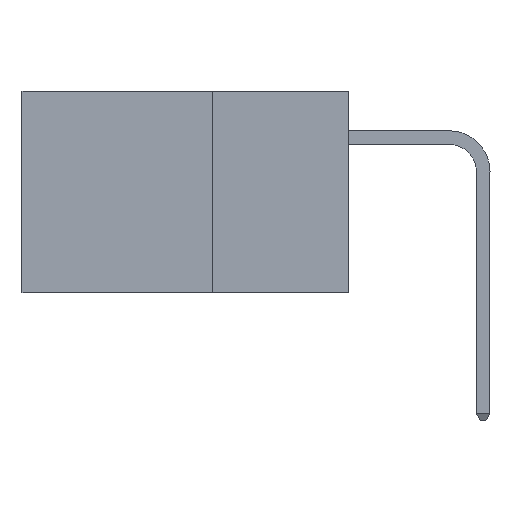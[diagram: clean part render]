
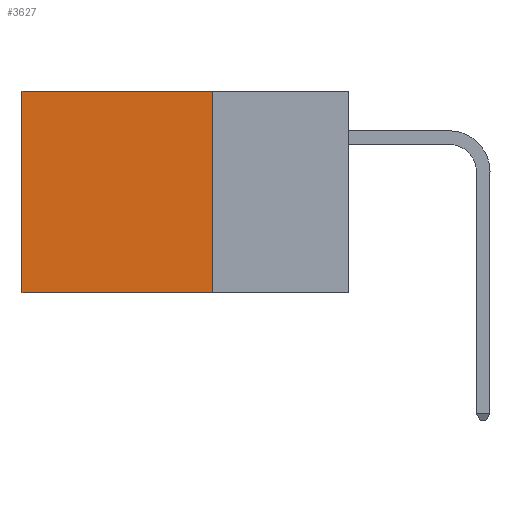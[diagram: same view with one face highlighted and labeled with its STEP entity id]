
A CAD part, left-side view. The second image highlights one B-rep face of the part: STEP entity #3627.
In plain terms, the highlighted planar face has unit normal (-1, 0, 0).
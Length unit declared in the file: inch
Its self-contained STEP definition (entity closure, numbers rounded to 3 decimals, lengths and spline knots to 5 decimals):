
#267 = VECTOR ( 'NONE', #10848, 39.37008 ) ;
#1266 = ORIENTED_EDGE ( 'NONE', *, *, #14544, .F. ) ;
#2196 = FACE_OUTER_BOUND ( 'NONE', #18392, .T. ) ;
#2317 = ORIENTED_EDGE ( 'NONE', *, *, #10987, .T. ) ;
#2890 = LINE ( 'NONE', #13136, #16023 ) ;
#3001 = LINE ( 'NONE', #18171, #267 ) ;
#3627 = ADVANCED_FACE ( 'NONE', ( #2196 ), #4721, .F. ) ;
#4330 = ORIENTED_EDGE ( 'NONE', *, *, #10571, .T. ) ;
#4341 = DIRECTION ( 'NONE',  ( 0., 1., 0. ) ) ;
#4394 = DIRECTION ( 'NONE',  ( 0., 0., -1. ) ) ;
#4463 = DIRECTION ( 'NONE',  ( 0., 0., -1. ) ) ;
#4721 = PLANE ( 'NONE',  #15591 ) ;
#5076 = VECTOR ( 'NONE', #12390, 39.37008 ) ;
#5554 = LINE ( 'NONE', #10924, #5076 ) ;
#6220 = CARTESIAN_POINT ( 'NONE',  ( 0.2875, 0.25, 0. ) ) ;
#6530 = ORIENTED_EDGE ( 'NONE', *, *, #11255, .F. ) ;
#10320 = VERTEX_POINT ( 'NONE', #18517 ) ;
#10571 = EDGE_CURVE ( 'NONE', #16939, #10320, #5554, .T. ) ;
#10848 = DIRECTION ( 'NONE',  ( 0., 0., -1. ) ) ;
#10924 = CARTESIAN_POINT ( 'NONE',  ( 0.2875, 0.25, 0. ) ) ;
#10987 = EDGE_CURVE ( 'NONE', #10320, #11083, #3001, .T. ) ;
#11083 = VERTEX_POINT ( 'NONE', #18299 ) ;
#11255 = EDGE_CURVE ( 'NONE', #16939, #12041, #17693, .T. ) ;
#11379 = CARTESIAN_POINT ( 'NONE',  ( 0.2875, 0.25, 0. ) ) ;
#12041 = VERTEX_POINT ( 'NONE', #12470 ) ;
#12390 = DIRECTION ( 'NONE',  ( 0., 1., 0. ) ) ;
#12470 = CARTESIAN_POINT ( 'NONE',  ( 0.2875, 0.25, -0.37 ) ) ;
#13131 = CARTESIAN_POINT ( 'NONE',  ( 0.2875, 0.25, 0. ) ) ;
#13136 = CARTESIAN_POINT ( 'NONE',  ( 0.2875, 0.25, -0.37 ) ) ;
#14544 = EDGE_CURVE ( 'NONE', #12041, #11083, #2890, .T. ) ;
#15432 = VECTOR ( 'NONE', #4394, 39.37008 ) ;
#15591 = AXIS2_PLACEMENT_3D ( 'NONE', #13131, #17648, #4463 ) ;
#16023 = VECTOR ( 'NONE', #4341, 39.37008 ) ;
#16939 = VERTEX_POINT ( 'NONE', #6220 ) ;
#17648 = DIRECTION ( 'NONE',  ( 1., 0., 0. ) ) ;
#17693 = LINE ( 'NONE', #11379, #15432 ) ;
#18171 = CARTESIAN_POINT ( 'NONE',  ( 0.2875, 0.6, 0. ) ) ;
#18299 = CARTESIAN_POINT ( 'NONE',  ( 0.2875, 0.6, -0.37 ) ) ;
#18392 = EDGE_LOOP ( 'NONE', ( #2317, #1266, #6530, #4330 ) ) ;
#18517 = CARTESIAN_POINT ( 'NONE',  ( 0.2875, 0.6, 0. ) ) ;
